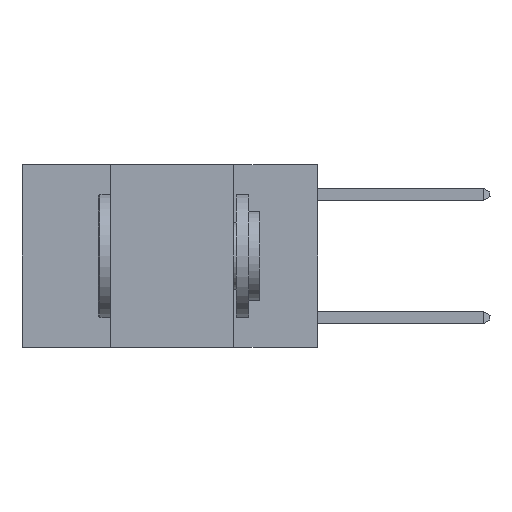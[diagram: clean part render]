
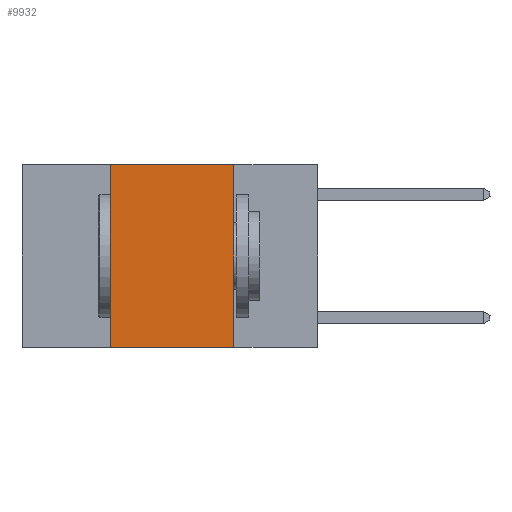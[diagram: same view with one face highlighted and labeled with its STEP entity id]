
A CAD part, left-side view. The second image highlights one B-rep face of the part: STEP entity #9932.
In plain terms, the highlighted planar face has unit normal (-1, 0, 0).
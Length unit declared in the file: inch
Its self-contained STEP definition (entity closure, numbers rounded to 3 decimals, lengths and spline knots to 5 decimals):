
#395 = VERTEX_POINT ( 'NONE', #4823 ) ;
#516 = PLANE ( 'NONE',  #4415 ) ;
#536 = CARTESIAN_POINT ( 'NONE',  ( 0., 0.17, -0.37 ) ) ;
#1002 = EDGE_CURVE ( 'NONE', #5173, #395, #9392, .T. ) ;
#1101 = EDGE_CURVE ( 'NONE', #395, #4724, #2869, .T. ) ;
#1220 = FACE_OUTER_BOUND ( 'NONE', #9349, .T. ) ;
#2163 = CARTESIAN_POINT ( 'NONE',  ( 0., 0.42, 0. ) ) ;
#2431 = VECTOR ( 'NONE', #5677, 39.37008 ) ;
#2869 = LINE ( 'NONE', #11388, #5941 ) ;
#3048 = DIRECTION ( 'NONE',  ( 0., 0., -1. ) ) ;
#3350 = CARTESIAN_POINT ( 'NONE',  ( 0., 0.6, 0. ) ) ;
#3529 = CARTESIAN_POINT ( 'NONE',  ( 0., 0.42, 0. ) ) ;
#3692 = EDGE_CURVE ( 'NONE', #11531, #5173, #11278, .T. ) ;
#3937 = CARTESIAN_POINT ( 'NONE',  ( 0., 0.6, -0.37 ) ) ;
#4004 = CARTESIAN_POINT ( 'NONE',  ( 0., 0.6, 0. ) ) ;
#4415 = AXIS2_PLACEMENT_3D ( 'NONE', #3350, #7176, #6155 ) ;
#4569 = DIRECTION ( 'NONE',  ( 0., -1., 0. ) ) ;
#4724 = VERTEX_POINT ( 'NONE', #536 ) ;
#4823 = CARTESIAN_POINT ( 'NONE',  ( 0., 0.17, 0. ) ) ;
#5173 = VERTEX_POINT ( 'NONE', #3529 ) ;
#5677 = DIRECTION ( 'NONE',  ( 0., -1., 0. ) ) ;
#5941 = VECTOR ( 'NONE', #3048, 39.37008 ) ;
#5963 = DIRECTION ( 'NONE',  ( 0., 0., 1. ) ) ;
#6155 = DIRECTION ( 'NONE',  ( 0., 0., -1. ) ) ;
#6264 = ORIENTED_EDGE ( 'NONE', *, *, #11950, .T. ) ;
#6415 = ORIENTED_EDGE ( 'NONE', *, *, #3692, .F. ) ;
#6473 = CARTESIAN_POINT ( 'NONE',  ( 0., 0.42, -0.37 ) ) ;
#7075 = ORIENTED_EDGE ( 'NONE', *, *, #1002, .F. ) ;
#7176 = DIRECTION ( 'NONE',  ( 1., 0., 0. ) ) ;
#8341 = VECTOR ( 'NONE', #4569, 39.37008 ) ;
#9349 = EDGE_LOOP ( 'NONE', ( #10551, #7075, #6415, #6264 ) ) ;
#9392 = LINE ( 'NONE', #4004, #2431 ) ;
#9932 = ADVANCED_FACE ( 'NONE', ( #1220 ), #516, .F. ) ;
#10122 = LINE ( 'NONE', #3937, #8341 ) ;
#10551 = ORIENTED_EDGE ( 'NONE', *, *, #1101, .F. ) ;
#11278 = LINE ( 'NONE', #2163, #11527 ) ;
#11388 = CARTESIAN_POINT ( 'NONE',  ( 0., 0.17, 0. ) ) ;
#11527 = VECTOR ( 'NONE', #5963, 39.37008 ) ;
#11531 = VERTEX_POINT ( 'NONE', #6473 ) ;
#11950 = EDGE_CURVE ( 'NONE', #11531, #4724, #10122, .T. ) ;
